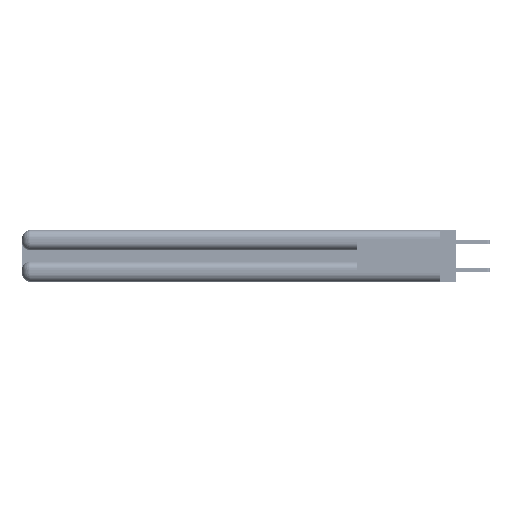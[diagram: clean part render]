
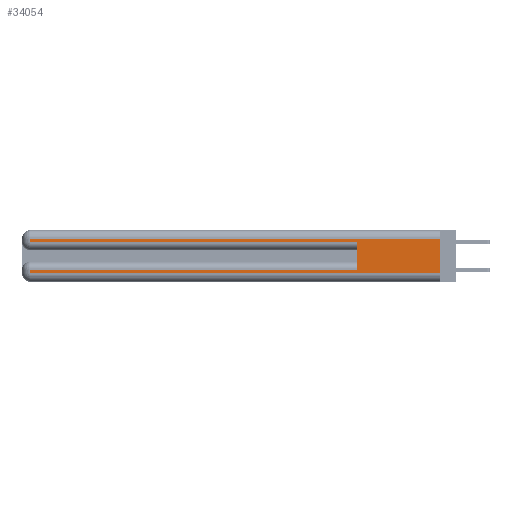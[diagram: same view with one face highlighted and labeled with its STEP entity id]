
A CAD part, left-side view. The second image highlights one B-rep face of the part: STEP entity #34054.
In plain terms, the highlighted planar face has unit normal (-1, 0, 0).
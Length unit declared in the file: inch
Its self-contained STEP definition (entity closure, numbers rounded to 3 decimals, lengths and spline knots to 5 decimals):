
#106 = VERTEX_POINT ( 'NONE', #30833 ) ;
#179 = DIRECTION ( 'NONE',  ( 0., -1., 0. ) ) ;
#597 = DIRECTION ( 'NONE',  ( 0., -1., 0. ) ) ;
#599 = CARTESIAN_POINT ( 'NONE',  ( 0., 0.6, 0.145 ) ) ;
#3661 = CARTESIAN_POINT ( 'NONE',  ( 0., 0., 0.37 ) ) ;
#4444 = LINE ( 'NONE', #34833, #11377 ) ;
#5952 = VERTEX_POINT ( 'NONE', #11866 ) ;
#7573 = CARTESIAN_POINT ( 'NONE',  ( 0., 0., 0.06 ) ) ;
#7795 = LINE ( 'NONE', #10428, #26451 ) ;
#7805 = CARTESIAN_POINT ( 'NONE',  ( 0., 0., 0.37 ) ) ;
#7904 = LINE ( 'NONE', #37042, #36675 ) ;
#7938 = PLANE ( 'NONE',  #10377 ) ;
#8651 = VECTOR ( 'NONE', #597, 39.37008 ) ;
#10307 = LINE ( 'NONE', #42006, #13508 ) ;
#10377 = AXIS2_PLACEMENT_3D ( 'NONE', #7805, #21083, #34772 ) ;
#10428 = CARTESIAN_POINT ( 'NONE',  ( 0., 0., 0.285 ) ) ;
#10846 = LINE ( 'NONE', #3661, #30029 ) ;
#11377 = VECTOR ( 'NONE', #38844, 39.37008 ) ;
#11619 = CARTESIAN_POINT ( 'NONE',  ( 0., 2.94, 0.06 ) ) ;
#11866 = CARTESIAN_POINT ( 'NONE',  ( 0., 2.94, 0.31 ) ) ;
#12605 = VECTOR ( 'NONE', #28274, 39.37008 ) ;
#13077 = EDGE_CURVE ( 'NONE', #106, #18923, #41594, .T. ) ;
#13418 = ORIENTED_EDGE ( 'NONE', *, *, #43778, .T. ) ;
#13508 = VECTOR ( 'NONE', #35154, 39.37008 ) ;
#14589 = CARTESIAN_POINT ( 'NONE',  ( 0., 2.94, 0.37 ) ) ;
#16398 = ORIENTED_EDGE ( 'NONE', *, *, #24358, .T. ) ;
#16815 = DIRECTION ( 'NONE',  ( 0., 0., -1. ) ) ;
#17768 = FACE_OUTER_BOUND ( 'NONE', #18288, .T. ) ;
#17868 = DIRECTION ( 'NONE',  ( 0., 0., 1. ) ) ;
#18288 = EDGE_LOOP ( 'NONE', ( #32025, #37418, #16398, #25095, #22047, #22901, #26190, #13418 ) ) ;
#18498 = EDGE_CURVE ( 'NONE', #23959, #22691, #7904, .T. ) ;
#18923 = VERTEX_POINT ( 'NONE', #36575 ) ;
#21083 = DIRECTION ( 'NONE',  ( 1., 0., 0. ) ) ;
#22047 = ORIENTED_EDGE ( 'NONE', *, *, #13077, .F. ) ;
#22083 = VERTEX_POINT ( 'NONE', #36946 ) ;
#22691 = VERTEX_POINT ( 'NONE', #11619 ) ;
#22901 = ORIENTED_EDGE ( 'NONE', *, *, #27360, .T. ) ;
#23959 = VERTEX_POINT ( 'NONE', #40102 ) ;
#24107 = EDGE_CURVE ( 'NONE', #39377, #18923, #7795, .T. ) ;
#24358 = EDGE_CURVE ( 'NONE', #5952, #39377, #39785, .T. ) ;
#25058 = VECTOR ( 'NONE', #17868, 39.37008 ) ;
#25095 = ORIENTED_EDGE ( 'NONE', *, *, #24107, .T. ) ;
#26190 = ORIENTED_EDGE ( 'NONE', *, *, #18498, .T. ) ;
#26451 = VECTOR ( 'NONE', #179, 39.37008 ) ;
#26560 = EDGE_CURVE ( 'NONE', #22083, #40066, #10846, .T. ) ;
#27360 = EDGE_CURVE ( 'NONE', #106, #23959, #10307, .T. ) ;
#27836 = LINE ( 'NONE', #41669, #8651 ) ;
#28274 = DIRECTION ( 'NONE',  ( 0., 0., -1. ) ) ;
#30029 = VECTOR ( 'NONE', #34339, 39.37008 ) ;
#30246 = CARTESIAN_POINT ( 'NONE',  ( 0., 2.94, 0.285 ) ) ;
#30833 = CARTESIAN_POINT ( 'NONE',  ( 0., 0.6, 0.085 ) ) ;
#32025 = ORIENTED_EDGE ( 'NONE', *, *, #26560, .F. ) ;
#34054 = ADVANCED_FACE ( 'NONE', ( #17768 ), #7938, .F. ) ;
#34339 = DIRECTION ( 'NONE',  ( 0., 0., -1. ) ) ;
#34772 = DIRECTION ( 'NONE',  ( 0., 0., -1. ) ) ;
#34833 = CARTESIAN_POINT ( 'NONE',  ( 0., 0., 0.31 ) ) ;
#35154 = DIRECTION ( 'NONE',  ( 0., 1., 0. ) ) ;
#36575 = CARTESIAN_POINT ( 'NONE',  ( 0., 0.6, 0.285 ) ) ;
#36675 = VECTOR ( 'NONE', #16815, 39.37008 ) ;
#36946 = CARTESIAN_POINT ( 'NONE',  ( 0., 0., 0.31 ) ) ;
#37042 = CARTESIAN_POINT ( 'NONE',  ( 0., 2.94, 0.37 ) ) ;
#37418 = ORIENTED_EDGE ( 'NONE', *, *, #40280, .T. ) ;
#38844 = DIRECTION ( 'NONE',  ( 0., 1., 0. ) ) ;
#39377 = VERTEX_POINT ( 'NONE', #30246 ) ;
#39785 = LINE ( 'NONE', #14589, #12605 ) ;
#40066 = VERTEX_POINT ( 'NONE', #7573 ) ;
#40102 = CARTESIAN_POINT ( 'NONE',  ( 0., 2.94, 0.085 ) ) ;
#40280 = EDGE_CURVE ( 'NONE', #22083, #5952, #4444, .T. ) ;
#41594 = LINE ( 'NONE', #599, #25058 ) ;
#41669 = CARTESIAN_POINT ( 'NONE',  ( 0., 0., 0.06 ) ) ;
#42006 = CARTESIAN_POINT ( 'NONE',  ( 0., 0., 0.085 ) ) ;
#43778 = EDGE_CURVE ( 'NONE', #22691, #40066, #27836, .T. ) ;
